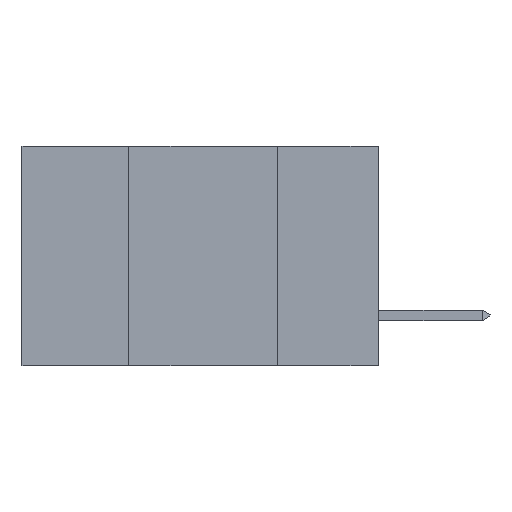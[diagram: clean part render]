
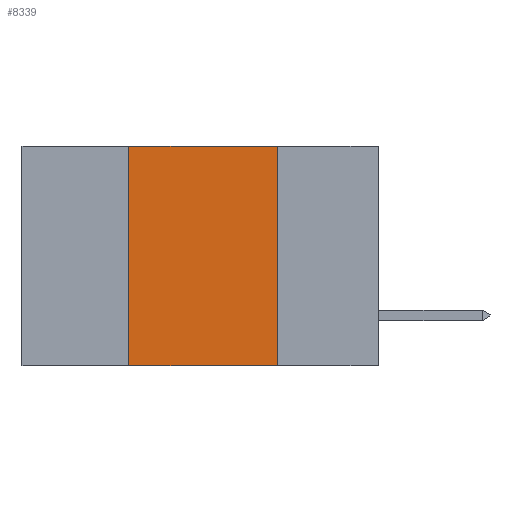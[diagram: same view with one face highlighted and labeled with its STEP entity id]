
A CAD part, left-side view. The second image highlights one B-rep face of the part: STEP entity #8339.
In plain terms, the highlighted planar face has unit normal (-1, 0, 0).
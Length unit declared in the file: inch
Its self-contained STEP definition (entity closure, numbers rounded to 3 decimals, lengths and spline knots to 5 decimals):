
#474 = ORIENTED_EDGE ( 'NONE', *, *, #8722, .F. ) ;
#543 = CARTESIAN_POINT ( 'NONE',  ( 0., 0.17, -0.37 ) ) ;
#663 = CARTESIAN_POINT ( 'NONE',  ( 0., 0.6, -0.37 ) ) ;
#1231 = VECTOR ( 'NONE', #8080, 39.37008 ) ;
#1652 = CARTESIAN_POINT ( 'NONE',  ( 0., 0.17, 0. ) ) ;
#1774 = EDGE_CURVE ( 'NONE', #9268, #2338, #3719, .T. ) ;
#1876 = DIRECTION ( 'NONE',  ( 0., 0., 1. ) ) ;
#1904 = VECTOR ( 'NONE', #8311, 39.37008 ) ;
#1975 = LINE ( 'NONE', #2691, #1231 ) ;
#2338 = VERTEX_POINT ( 'NONE', #543 ) ;
#2468 = ORIENTED_EDGE ( 'NONE', *, *, #3644, .F. ) ;
#2691 = CARTESIAN_POINT ( 'NONE',  ( 0., 0.6, 0. ) ) ;
#3101 = CARTESIAN_POINT ( 'NONE',  ( 0., 0.42, -0.37 ) ) ;
#3124 = PLANE ( 'NONE',  #8749 ) ;
#3324 = CARTESIAN_POINT ( 'NONE',  ( 0., 0.42, 0. ) ) ;
#3644 = EDGE_CURVE ( 'NONE', #3846, #2338, #5549, .T. ) ;
#3719 = LINE ( 'NONE', #663, #1904 ) ;
#3846 = VERTEX_POINT ( 'NONE', #1652 ) ;
#4621 = CARTESIAN_POINT ( 'NONE',  ( 0., 0.17, 0. ) ) ;
#4744 = FACE_OUTER_BOUND ( 'NONE', #4749, .T. ) ;
#4749 = EDGE_LOOP ( 'NONE', ( #2468, #9540, #474, #9815 ) ) ;
#5458 = DIRECTION ( 'NONE',  ( 0., 0., -1. ) ) ;
#5549 = LINE ( 'NONE', #4621, #6888 ) ;
#5560 = DIRECTION ( 'NONE',  ( 0., 0., -1. ) ) ;
#6353 = CARTESIAN_POINT ( 'NONE',  ( 0., 0.42, 0. ) ) ;
#6888 = VECTOR ( 'NONE', #5458, 39.37008 ) ;
#7019 = LINE ( 'NONE', #3324, #8959 ) ;
#8080 = DIRECTION ( 'NONE',  ( 0., -1., 0. ) ) ;
#8215 = EDGE_CURVE ( 'NONE', #8475, #3846, #1975, .T. ) ;
#8311 = DIRECTION ( 'NONE',  ( 0., -1., 0. ) ) ;
#8339 = ADVANCED_FACE ( 'NONE', ( #4744 ), #3124, .F. ) ;
#8475 = VERTEX_POINT ( 'NONE', #6353 ) ;
#8716 = CARTESIAN_POINT ( 'NONE',  ( 0., 0.6, 0. ) ) ;
#8722 = EDGE_CURVE ( 'NONE', #9268, #8475, #7019, .T. ) ;
#8749 = AXIS2_PLACEMENT_3D ( 'NONE', #8716, #9366, #5560 ) ;
#8959 = VECTOR ( 'NONE', #1876, 39.37008 ) ;
#9268 = VERTEX_POINT ( 'NONE', #3101 ) ;
#9366 = DIRECTION ( 'NONE',  ( 1., 0., 0. ) ) ;
#9540 = ORIENTED_EDGE ( 'NONE', *, *, #8215, .F. ) ;
#9815 = ORIENTED_EDGE ( 'NONE', *, *, #1774, .T. ) ;
